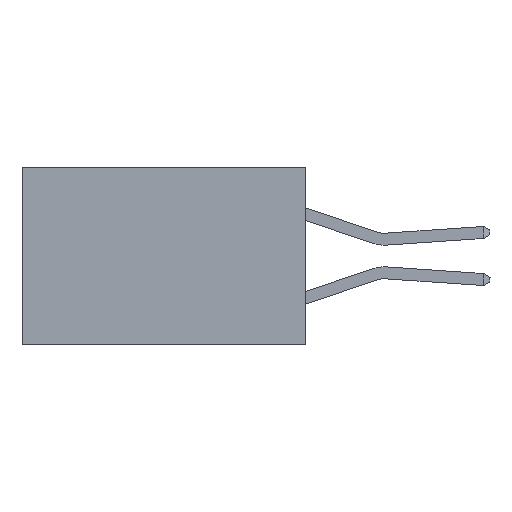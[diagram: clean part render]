
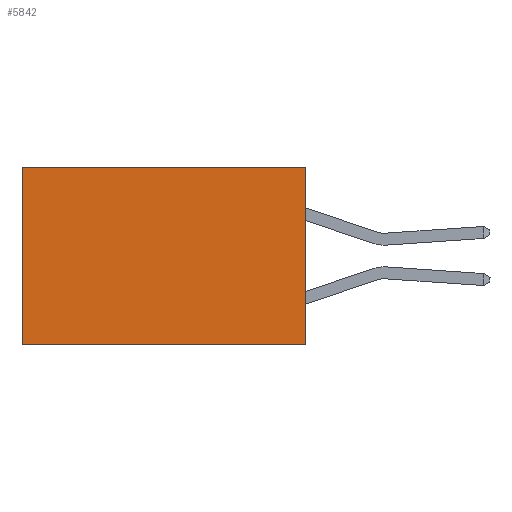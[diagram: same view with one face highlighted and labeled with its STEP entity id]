
A CAD part, left-side view. The second image highlights one B-rep face of the part: STEP entity #5842.
In plain terms, the highlighted planar face has unit normal (-1, 0, 0).
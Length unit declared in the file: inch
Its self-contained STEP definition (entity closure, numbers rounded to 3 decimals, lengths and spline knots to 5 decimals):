
#662 = CARTESIAN_POINT ( 'NONE',  ( 0.277, 0.59, 0. ) ) ;
#903 = VECTOR ( 'NONE', #5304, 39.37008 ) ;
#1846 = CARTESIAN_POINT ( 'NONE',  ( 0.277, 0.59, -0.37 ) ) ;
#2321 = VERTEX_POINT ( 'NONE', #1846 ) ;
#2396 = VECTOR ( 'NONE', #6315, 39.37008 ) ;
#2436 = PLANE ( 'NONE',  #4255 ) ;
#2709 = ORIENTED_EDGE ( 'NONE', *, *, #4104, .F. ) ;
#2951 = DIRECTION ( 'NONE',  ( 0., 1., 0. ) ) ;
#3041 = CARTESIAN_POINT ( 'NONE',  ( 0.277, 0., -0.37 ) ) ;
#3131 = EDGE_CURVE ( 'NONE', #4852, #7685, #6958, .T. ) ;
#3153 = CARTESIAN_POINT ( 'NONE',  ( 0.277, 0., -0.37 ) ) ;
#3254 = EDGE_CURVE ( 'NONE', #7685, #2321, #7024, .T. ) ;
#3256 = LINE ( 'NONE', #3041, #6269 ) ;
#3833 = ORIENTED_EDGE ( 'NONE', *, *, #3131, .T. ) ;
#3857 = DIRECTION ( 'NONE',  ( 0., 0., -1. ) ) ;
#3925 = EDGE_LOOP ( 'NONE', ( #6555, #2709, #7216, #3833 ) ) ;
#4104 = EDGE_CURVE ( 'NONE', #4735, #2321, #3256, .T. ) ;
#4116 = EDGE_CURVE ( 'NONE', #4852, #4735, #4689, .T. ) ;
#4255 = AXIS2_PLACEMENT_3D ( 'NONE', #3153, #7057, #3857 ) ;
#4476 = FACE_OUTER_BOUND ( 'NONE', #3925, .T. ) ;
#4522 = CARTESIAN_POINT ( 'NONE',  ( 0.277, 0., 0. ) ) ;
#4689 = LINE ( 'NONE', #5238, #903 ) ;
#4735 = VERTEX_POINT ( 'NONE', #7253 ) ;
#4852 = VERTEX_POINT ( 'NONE', #7046 ) ;
#5238 = CARTESIAN_POINT ( 'NONE',  ( 0.277, 0., -0.37 ) ) ;
#5304 = DIRECTION ( 'NONE',  ( 0., 0., -1. ) ) ;
#5742 = VECTOR ( 'NONE', #7153, 39.37008 ) ;
#5828 = CARTESIAN_POINT ( 'NONE',  ( 0.277, 0.59, -0.37 ) ) ;
#5842 = ADVANCED_FACE ( 'NONE', ( #4476 ), #2436, .F. ) ;
#6269 = VECTOR ( 'NONE', #2951, 39.37008 ) ;
#6315 = DIRECTION ( 'NONE',  ( 0., 0., -1. ) ) ;
#6555 = ORIENTED_EDGE ( 'NONE', *, *, #3254, .T. ) ;
#6958 = LINE ( 'NONE', #4522, #5742 ) ;
#7024 = LINE ( 'NONE', #5828, #2396 ) ;
#7046 = CARTESIAN_POINT ( 'NONE',  ( 0.277, 0., 0. ) ) ;
#7057 = DIRECTION ( 'NONE',  ( 1., 0., 0. ) ) ;
#7153 = DIRECTION ( 'NONE',  ( 0., 1., 0. ) ) ;
#7216 = ORIENTED_EDGE ( 'NONE', *, *, #4116, .F. ) ;
#7253 = CARTESIAN_POINT ( 'NONE',  ( 0.277, 0., -0.37 ) ) ;
#7685 = VERTEX_POINT ( 'NONE', #662 ) ;
